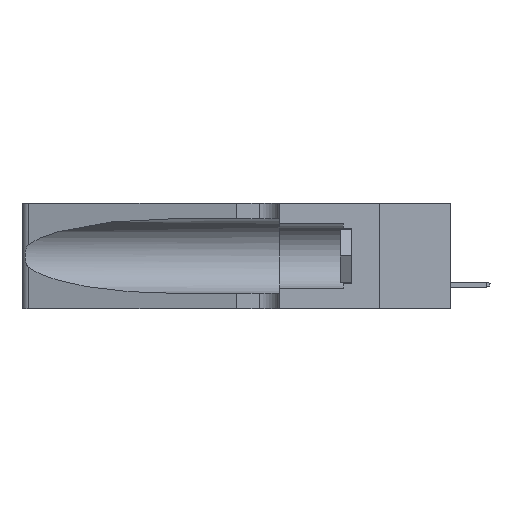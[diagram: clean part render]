
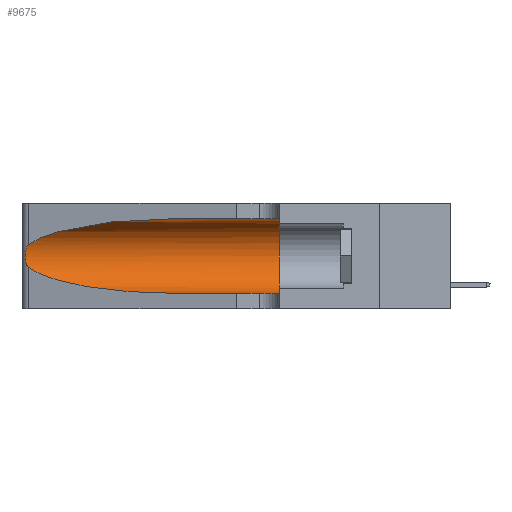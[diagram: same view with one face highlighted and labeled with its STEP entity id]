
A CAD part, left-side view. The second image highlights one B-rep face of the part: STEP entity #9675.
In plain terms, the highlighted cylindrical face has radius 3.308 mm (diameter 6.617 mm), a partial arc.
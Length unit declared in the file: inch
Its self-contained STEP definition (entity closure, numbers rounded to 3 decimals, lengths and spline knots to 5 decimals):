
#135 = ORIENTED_EDGE ( 'NONE', *, *, #3179, .F. ) ;
#507 = CARTESIAN_POINT ( 'NONE',  ( 0.25787, 1.23484, 0.2124 ) ) ;
#1126 = CARTESIAN_POINT ( 'NONE',  ( 0.1305, 0.35, 0.185 ) ) ;
#1593 = EDGE_CURVE ( 'NONE', #7048, #37222, #31382, .T. ) ;
#1693 = CARTESIAN_POINT ( 'NONE',  ( 0.25856, 1.23593, 0.16098 ) ) ;
#3179 = EDGE_CURVE ( 'NONE', #10332, #4263, #31605, .T. ) ;
#3878 = CARTESIAN_POINT ( 'NONE',  ( 0.2373, 1.15595, 0.08982 ) ) ;
#4176 = DIRECTION ( 'NONE',  ( 0., 0., 1. ) ) ;
#4263 = VERTEX_POINT ( 'NONE', #32987 ) ;
#6588 = CARTESIAN_POINT ( 'NONE',  ( 0.25487, 1.22718, 0.22369 ) ) ;
#6670 = DIRECTION ( 'NONE',  ( 0., 0., -1. ) ) ;
#6725 = CARTESIAN_POINT ( 'NONE',  ( 0.1305, 0.72297, 0.05475 ) ) ;
#6789 = CARTESIAN_POINT ( 'NONE',  ( 0.1305, 1.61858, 0.05475 ) ) ;
#7048 = VERTEX_POINT ( 'NONE', #37167 ) ;
#7579 = CARTESIAN_POINT ( 'NONE',  ( 0.26075, 1.23896, 0.19203 ) ) ;
#9375 = CARTESIAN_POINT ( 'NONE',  ( 0.25487, 1.22718, 0.14631 ) ) ;
#9675 = ADVANCED_FACE ( 'NONE', ( #13162 ), #15988, .F. ) ;
#10332 = VERTEX_POINT ( 'NONE', #14253 ) ;
#12117 = B_SPLINE_CURVE_WITH_KNOTS ( 'NONE', 3,
 ( #6588, #31280, #15911, #507, #37557, #32270, #7579, #14065, #13665, #1693, #23556, #32475, #26006, #17117 ),
 .UNSPECIFIED., .F., .F.,
 ( 4, 2, 2, 2, 2, 2, 4 ),
 ( 0., 0.00027, 0.00053, 0.00107, 0.0016, 0.00187, 0.00214 ),
 .UNSPECIFIED. ) ;
#12295 = CARTESIAN_POINT ( 'NONE',  ( 0.1305, 0.72297, 0.31525 ) ) ;
#13162 = FACE_OUTER_BOUND ( 'NONE', #29796, .T. ) ;
#13665 = CARTESIAN_POINT ( 'NONE',  ( 0.26017, 1.23833, 0.17102 ) ) ;
#13783 = ORIENTED_EDGE ( 'NONE', *, *, #19406, .F. ) ;
#14065 = CARTESIAN_POINT ( 'NONE',  ( 0.26075, 1.23896, 0.178 ) ) ;
#14253 = CARTESIAN_POINT ( 'NONE',  ( 0.1305, 0.35, 0.31525 ) ) ;
#14834 = AXIS2_PLACEMENT_3D ( 'NONE', #1126, #37984, #4176 ) ;
#15134 = EDGE_CURVE ( 'NONE', #25103, #7048, #12117, .T. ) ;
#15525 = CARTESIAN_POINT ( 'NONE',  ( 0.18966, 0.96281, 0.31525 ) ) ;
#15820 = ORIENTED_EDGE ( 'NONE', *, *, #15134, .T. ) ;
#15911 = CARTESIAN_POINT ( 'NONE',  ( 0.25639, 1.23184, 0.21858 ) ) ;
#15988 = CYLINDRICAL_SURFACE ( 'NONE', #19613, 0.13025 ) ;
#16195 = VERTEX_POINT ( 'NONE', #33573 ) ;
#16298 = LINE ( 'NONE', #6789, #35156 ) ;
#16733 = EDGE_CURVE ( 'NONE', #16195, #25103, #30320, .T. ) ;
#17117 = CARTESIAN_POINT ( 'NONE',  ( 0.25487, 1.22718, 0.14631 ) ) ;
#18454 = ORIENTED_EDGE ( 'NONE', *, *, #16733, .T. ) ;
#19406 = EDGE_CURVE ( 'NONE', #16195, #10332, #39170, .T. ) ;
#19613 = AXIS2_PLACEMENT_3D ( 'NONE', #24689, #28325, #6670 ) ;
#20332 = DIRECTION ( 'NONE',  ( 0., -1., 0. ) ) ;
#23319 = ORIENTED_EDGE ( 'NONE', *, *, #37696, .T. ) ;
#23556 = CARTESIAN_POINT ( 'NONE',  ( 0.25789, 1.23486, 0.15765 ) ) ;
#24309 = CARTESIAN_POINT ( 'NONE',  ( 0.1305, 1.61858, 0.31525 ) ) ;
#24689 = CARTESIAN_POINT ( 'NONE',  ( 0.1305, 1.61858, 0.185 ) ) ;
#25103 = VERTEX_POINT ( 'NONE', #36559 ) ;
#26006 = CARTESIAN_POINT ( 'NONE',  ( 0.25555, 1.22993, 0.14849 ) ) ;
#28325 = DIRECTION ( 'NONE',  ( 0., -1., 0. ) ) ;
#28875 = CARTESIAN_POINT ( 'NONE',  ( 0.1305, 0.72297, 0.05475 ) ) ;
#29028 = ORIENTED_EDGE ( 'NONE', *, *, #1593, .T. ) ;
#29796 = EDGE_LOOP ( 'NONE', ( #18454, #15820, #29028, #23319, #135, #13783 ) ) ;
#30320 =( BOUNDED_CURVE ( )  B_SPLINE_CURVE ( 3, ( #12295, #15525, #36749, #37158 ),
 .UNSPECIFIED., .F., .F. ) 
 B_SPLINE_CURVE_WITH_KNOTS ( ( 4, 4 ),
 ( 1.5708, 2.84003 ),
 .UNSPECIFIED. ) 
 CURVE ( )  GEOMETRIC_REPRESENTATION_ITEM ( )  RATIONAL_B_SPLINE_CURVE ( ( 1., 0.87, 0.87, 1. ) ) 
 REPRESENTATION_ITEM ( '' )  );
#31280 = CARTESIAN_POINT ( 'NONE',  ( 0.25555, 1.22994, 0.2215 ) ) ;
#31382 =( BOUNDED_CURVE ( )  B_SPLINE_CURVE ( 3, ( #9375, #3878, #31611, #6725 ),
 .UNSPECIFIED., .F., .F. ) 
 B_SPLINE_CURVE_WITH_KNOTS ( ( 4, 4 ),
 ( 3.44316, 4.71239 ),
 .UNSPECIFIED. ) 
 CURVE ( )  GEOMETRIC_REPRESENTATION_ITEM ( )  RATIONAL_B_SPLINE_CURVE ( ( 1., 0.87, 0.87, 1. ) ) 
 REPRESENTATION_ITEM ( '' )  );
#31470 = DIRECTION ( 'NONE',  ( 0., -1., 0. ) ) ;
#31605 = CIRCLE ( 'NONE', #14834, 0.13025 ) ;
#31611 = CARTESIAN_POINT ( 'NONE',  ( 0.18966, 0.96281, 0.05475 ) ) ;
#32270 = CARTESIAN_POINT ( 'NONE',  ( 0.26018, 1.23835, 0.19895 ) ) ;
#32475 = CARTESIAN_POINT ( 'NONE',  ( 0.25639, 1.23186, 0.15144 ) ) ;
#32987 = CARTESIAN_POINT ( 'NONE',  ( 0.1305, 0.35, 0.05475 ) ) ;
#33573 = CARTESIAN_POINT ( 'NONE',  ( 0.1305, 0.72297, 0.31525 ) ) ;
#35156 = VECTOR ( 'NONE', #31470, 39.37008 ) ;
#35565 = VECTOR ( 'NONE', #20332, 39.37008 ) ;
#36559 = CARTESIAN_POINT ( 'NONE',  ( 0.25487, 1.22718, 0.22369 ) ) ;
#36749 = CARTESIAN_POINT ( 'NONE',  ( 0.2373, 1.15595, 0.28018 ) ) ;
#37158 = CARTESIAN_POINT ( 'NONE',  ( 0.25487, 1.22718, 0.22369 ) ) ;
#37167 = CARTESIAN_POINT ( 'NONE',  ( 0.25487, 1.22718, 0.14631 ) ) ;
#37222 = VERTEX_POINT ( 'NONE', #28875 ) ;
#37557 = CARTESIAN_POINT ( 'NONE',  ( 0.25854, 1.2359, 0.20912 ) ) ;
#37696 = EDGE_CURVE ( 'NONE', #37222, #4263, #16298, .T. ) ;
#37984 = DIRECTION ( 'NONE',  ( 0., 1., 0. ) ) ;
#39170 = LINE ( 'NONE', #24309, #35565 ) ;
